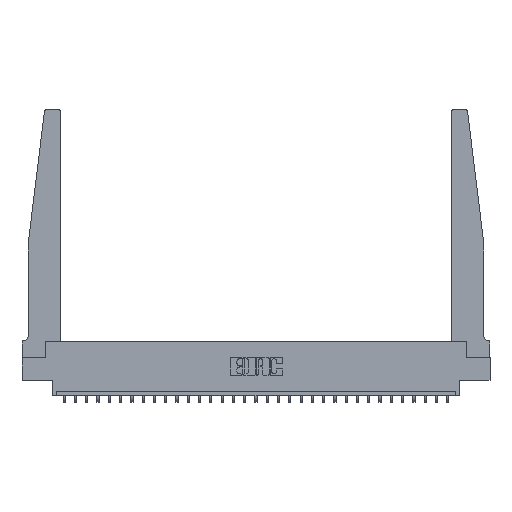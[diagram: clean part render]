
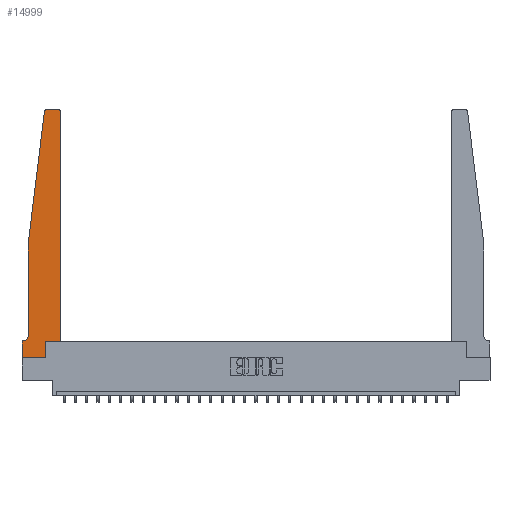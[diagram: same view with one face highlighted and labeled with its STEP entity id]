
A CAD part, top view. The second image highlights one B-rep face of the part: STEP entity #14999.
In plain terms, the highlighted planar face has unit normal (0, 0, 1).
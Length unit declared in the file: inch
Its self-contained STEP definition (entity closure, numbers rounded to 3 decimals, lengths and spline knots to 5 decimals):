
#154 = VECTOR ( 'NONE', #24299, 39.37008 ) ;
#228 = ORIENTED_EDGE ( 'NONE', *, *, #10893, .T. ) ;
#687 = DIRECTION ( 'NONE',  ( 0., 1., 0. ) ) ;
#1246 = LINE ( 'NONE', #5664, #19778 ) ;
#2255 = DIRECTION ( 'NONE',  ( 0., 0., 1. ) ) ;
#2275 = CIRCLE ( 'NONE', #5921, 0.03 ) ;
#2446 = CARTESIAN_POINT ( 'NONE',  ( 0.2605, 0.18, 0.37 ) ) ;
#3166 = LINE ( 'NONE', #20024, #154 ) ;
#3201 = VECTOR ( 'NONE', #22148, 39.37008 ) ;
#3552 = CIRCLE ( 'NONE', #19375, 0.03 ) ;
#3799 = CARTESIAN_POINT ( 'NONE',  ( 0.065, 1.25, 0.37 ) ) ;
#4984 = VECTOR ( 'NONE', #12653, 39.37008 ) ;
#5147 = VECTOR ( 'NONE', #12453, 39.37008 ) ;
#5467 = DIRECTION ( 'NONE',  ( 0., 1., 0. ) ) ;
#5502 = VERTEX_POINT ( 'NONE', #12891 ) ;
#5664 = CARTESIAN_POINT ( 'NONE',  ( 0.425, 0.18, 0.37 ) ) ;
#5921 = AXIS2_PLACEMENT_3D ( 'NONE', #13069, #2255, #6817 ) ;
#6069 = DIRECTION ( 'NONE',  ( -1., 0., 0. ) ) ;
#6717 = CARTESIAN_POINT ( 'NONE',  ( 0., 0., 0.37 ) ) ;
#6817 = DIRECTION ( 'NONE',  ( 1., 0., 0. ) ) ;
#7027 = DIRECTION ( 'NONE',  ( 0., 0., -1. ) ) ;
#7044 = VERTEX_POINT ( 'NONE', #2446 ) ;
#7159 = EDGE_CURVE ( 'NONE', #5502, #14416, #25851, .T. ) ;
#8183 = EDGE_CURVE ( 'NONE', #15478, #21306, #2275, .T. ) ;
#8313 = ORIENTED_EDGE ( 'NONE', *, *, #7159, .T. ) ;
#8324 = EDGE_CURVE ( 'NONE', #11562, #27978, #20282, .T. ) ;
#8713 = ORIENTED_EDGE ( 'NONE', *, *, #17567, .T. ) ;
#9197 = EDGE_LOOP ( 'NONE', ( #25192, #16405, #228, #12937, #21380, #10715, #8313, #13351, #24718, #16035, #8713, #22779 ) ) ;
#9698 = CARTESIAN_POINT ( 'NONE',  ( 0.2605, 0.18, 0.37 ) ) ;
#10060 = CARTESIAN_POINT ( 'NONE',  ( 0.015, 0.1875, 0.37 ) ) ;
#10140 = FACE_OUTER_BOUND ( 'NONE', #9197, .T. ) ;
#10538 = DIRECTION ( 'NONE',  ( 1., 0., 0. ) ) ;
#10715 = ORIENTED_EDGE ( 'NONE', *, *, #18786, .T. ) ;
#10893 = EDGE_CURVE ( 'NONE', #15096, #11562, #18671, .T. ) ;
#10919 = CARTESIAN_POINT ( 'NONE',  ( 0.425, 2.72, 0.37 ) ) ;
#11562 = VERTEX_POINT ( 'NONE', #22203 ) ;
#11957 = DIRECTION ( 'NONE',  ( -1., 0., 0. ) ) ;
#12099 = DIRECTION ( 'NONE',  ( -1., 0., 0. ) ) ;
#12453 = DIRECTION ( 'NONE',  ( 1., 0., 0. ) ) ;
#12653 = DIRECTION ( 'NONE',  ( 0., -1., 0. ) ) ;
#12795 = VERTEX_POINT ( 'NONE', #22146 ) ;
#12824 = DIRECTION ( 'NONE',  ( 0., 0., 1. ) ) ;
#12867 = EDGE_CURVE ( 'NONE', #7044, #24655, #16436, .T. ) ;
#12891 = CARTESIAN_POINT ( 'NONE',  ( 0., 0.1875, 0.37 ) ) ;
#12937 = ORIENTED_EDGE ( 'NONE', *, *, #8324, .T. ) ;
#13069 = CARTESIAN_POINT ( 'NONE',  ( 0.395, 2.72, 0.37 ) ) ;
#13351 = ORIENTED_EDGE ( 'NONE', *, *, #14543, .T. ) ;
#14227 = DIRECTION ( 'NONE',  ( 0., 0., 1. ) ) ;
#14416 = VERTEX_POINT ( 'NONE', #6717 ) ;
#14534 = CARTESIAN_POINT ( 'NONE',  ( 0., 0.1875, 0.37 ) ) ;
#14543 = EDGE_CURVE ( 'NONE', #14416, #12795, #3166, .T. ) ;
#14758 = VECTOR ( 'NONE', #11957, 39.37008 ) ;
#14775 = CARTESIAN_POINT ( 'NONE',  ( 0.25, 2.75, 0.37 ) ) ;
#14999 = ADVANCED_FACE ( 'NONE', ( #10140 ), #23316, .T. ) ;
#15096 = VERTEX_POINT ( 'NONE', #19884 ) ;
#15280 = CIRCLE ( 'NONE', #20270, 0.05 ) ;
#15478 = VERTEX_POINT ( 'NONE', #10919 ) ;
#16035 = ORIENTED_EDGE ( 'NONE', *, *, #12867, .T. ) ;
#16263 = DIRECTION ( 'NONE',  ( -0.122, -0.992, 0. ) ) ;
#16405 = ORIENTED_EDGE ( 'NONE', *, *, #23721, .T. ) ;
#16436 = LINE ( 'NONE', #25399, #5147 ) ;
#16869 = VECTOR ( 'NONE', #16263, 39.37008 ) ;
#17567 = EDGE_CURVE ( 'NONE', #24655, #15478, #1246, .T. ) ;
#17905 = EDGE_CURVE ( 'NONE', #12795, #7044, #24909, .T. ) ;
#17919 = VECTOR ( 'NONE', #12099, 39.37008 ) ;
#18413 = CARTESIAN_POINT ( 'NONE',  ( 0.065, 1.25, 0.37 ) ) ;
#18552 = CARTESIAN_POINT ( 'NONE',  ( 0.27653, 2.75, 0.37 ) ) ;
#18671 = LINE ( 'NONE', #3799, #16869 ) ;
#18786 = EDGE_CURVE ( 'NONE', #23133, #5502, #21192, .T. ) ;
#19375 = AXIS2_PLACEMENT_3D ( 'NONE', #23407, #14227, #21292 ) ;
#19640 = CARTESIAN_POINT ( 'NONE',  ( 0.015, 0.2375, 0.37 ) ) ;
#19778 = VECTOR ( 'NONE', #687, 39.37008 ) ;
#19832 = CARTESIAN_POINT ( 'NONE',  ( 0.425, 0.18, 0.37 ) ) ;
#19884 = CARTESIAN_POINT ( 'NONE',  ( 0.24675, 2.72367, 0.37 ) ) ;
#20024 = CARTESIAN_POINT ( 'NONE',  ( 0., 0., 0.37 ) ) ;
#20270 = AXIS2_PLACEMENT_3D ( 'NONE', #19640, #7027, #6069 ) ;
#20282 = LINE ( 'NONE', #18413, #3201 ) ;
#20558 = VERTEX_POINT ( 'NONE', #18552 ) ;
#21095 = EDGE_CURVE ( 'NONE', #21306, #20558, #25307, .T. ) ;
#21192 = LINE ( 'NONE', #23434, #17919 ) ;
#21292 = DIRECTION ( 'NONE',  ( 1., 0., 0. ) ) ;
#21306 = VERTEX_POINT ( 'NONE', #27442 ) ;
#21380 = ORIENTED_EDGE ( 'NONE', *, *, #23240, .T. ) ;
#22146 = CARTESIAN_POINT ( 'NONE',  ( 0.2605, 0., 0.37 ) ) ;
#22148 = DIRECTION ( 'NONE',  ( 0., -1., 0. ) ) ;
#22203 = CARTESIAN_POINT ( 'NONE',  ( 0.065, 1.25, 0.37 ) ) ;
#22779 = ORIENTED_EDGE ( 'NONE', *, *, #8183, .T. ) ;
#23133 = VERTEX_POINT ( 'NONE', #10060 ) ;
#23240 = EDGE_CURVE ( 'NONE', #27978, #23133, #15280, .T. ) ;
#23316 = PLANE ( 'NONE',  #24700 ) ;
#23407 = CARTESIAN_POINT ( 'NONE',  ( 0.27653, 2.72, 0.37 ) ) ;
#23434 = CARTESIAN_POINT ( 'NONE',  ( 0.065, 0.1875, 0.37 ) ) ;
#23721 = EDGE_CURVE ( 'NONE', #20558, #15096, #3552, .T. ) ;
#24299 = DIRECTION ( 'NONE',  ( 1., 0., 0. ) ) ;
#24655 = VERTEX_POINT ( 'NONE', #19832 ) ;
#24700 = AXIS2_PLACEMENT_3D ( 'NONE', #14534, #12824, #10538 ) ;
#24718 = ORIENTED_EDGE ( 'NONE', *, *, #17905, .T. ) ;
#24909 = LINE ( 'NONE', #9698, #27986 ) ;
#25192 = ORIENTED_EDGE ( 'NONE', *, *, #21095, .T. ) ;
#25201 = CARTESIAN_POINT ( 'NONE',  ( 0.065, 0.2375, 0.37 ) ) ;
#25307 = LINE ( 'NONE', #14775, #14758 ) ;
#25399 = CARTESIAN_POINT ( 'NONE',  ( 0.425, 0.18, 0.37 ) ) ;
#25724 = CARTESIAN_POINT ( 'NONE',  ( 0., 0., 0.37 ) ) ;
#25851 = LINE ( 'NONE', #25724, #4984 ) ;
#27442 = CARTESIAN_POINT ( 'NONE',  ( 0.395, 2.75, 0.37 ) ) ;
#27978 = VERTEX_POINT ( 'NONE', #25201 ) ;
#27986 = VECTOR ( 'NONE', #5467, 39.37008 ) ;
